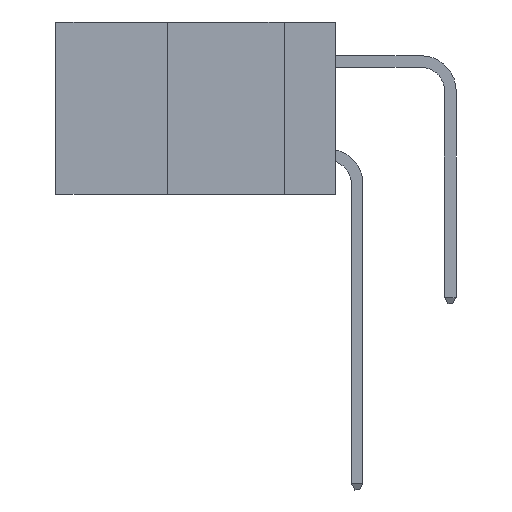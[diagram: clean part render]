
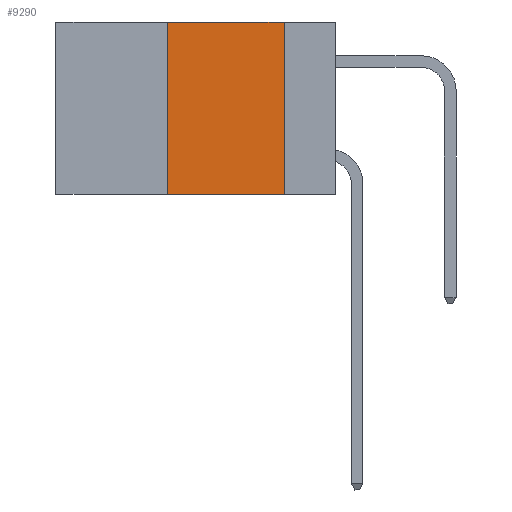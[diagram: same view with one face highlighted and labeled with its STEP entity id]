
A CAD part, left-side view. The second image highlights one B-rep face of the part: STEP entity #9290.
In plain terms, the highlighted planar face has unit normal (-1, 0, 0).
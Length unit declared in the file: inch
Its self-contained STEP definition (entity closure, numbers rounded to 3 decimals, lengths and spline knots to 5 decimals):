
#184 = ORIENTED_EDGE ( 'NONE', *, *, #9923, .F. ) ;
#198 = ORIENTED_EDGE ( 'NONE', *, *, #2164, .T. ) ;
#483 = CARTESIAN_POINT ( 'NONE',  ( 0., 0.36, -0.37 ) ) ;
#531 = LINE ( 'NONE', #1199, #10162 ) ;
#1199 = CARTESIAN_POINT ( 'NONE',  ( 0., 0.11, 0. ) ) ;
#1274 = DIRECTION ( 'NONE',  ( 0., 0., -1. ) ) ;
#1278 = VERTEX_POINT ( 'NONE', #7535 ) ;
#1319 = LINE ( 'NONE', #3607, #6776 ) ;
#1543 = DIRECTION ( 'NONE',  ( 1., 0., 0. ) ) ;
#1597 = EDGE_CURVE ( 'NONE', #6915, #7989, #531, .T. ) ;
#1694 = CARTESIAN_POINT ( 'NONE',  ( 0., 0.11, -0.37 ) ) ;
#2164 = EDGE_CURVE ( 'NONE', #4565, #7989, #7359, .T. ) ;
#2437 = VECTOR ( 'NONE', #5425, 39.37008 ) ;
#2674 = ORIENTED_EDGE ( 'NONE', *, *, #4798, .F. ) ;
#2956 = VECTOR ( 'NONE', #10733, 39.37008 ) ;
#3059 = CARTESIAN_POINT ( 'NONE',  ( 0., 0.6, 0. ) ) ;
#3607 = CARTESIAN_POINT ( 'NONE',  ( 0., 0.36, 0. ) ) ;
#4565 = VERTEX_POINT ( 'NONE', #483 ) ;
#4798 = EDGE_CURVE ( 'NONE', #1278, #6915, #9361, .T. ) ;
#5425 = DIRECTION ( 'NONE',  ( 0., -1., 0. ) ) ;
#6776 = VECTOR ( 'NONE', #7130, 39.37008 ) ;
#6915 = VERTEX_POINT ( 'NONE', #11232 ) ;
#7004 = CARTESIAN_POINT ( 'NONE',  ( 0., 0.6, 0. ) ) ;
#7130 = DIRECTION ( 'NONE',  ( 0., 0., 1. ) ) ;
#7359 = LINE ( 'NONE', #10716, #2956 ) ;
#7491 = EDGE_LOOP ( 'NONE', ( #9101, #2674, #184, #198 ) ) ;
#7535 = CARTESIAN_POINT ( 'NONE',  ( 0., 0.36, 0. ) ) ;
#7850 = DIRECTION ( 'NONE',  ( 0., 0., -1. ) ) ;
#7989 = VERTEX_POINT ( 'NONE', #1694 ) ;
#8117 = FACE_OUTER_BOUND ( 'NONE', #7491, .T. ) ;
#9101 = ORIENTED_EDGE ( 'NONE', *, *, #1597, .F. ) ;
#9290 = ADVANCED_FACE ( 'NONE', ( #8117 ), #11034, .F. ) ;
#9361 = LINE ( 'NONE', #3059, #2437 ) ;
#9923 = EDGE_CURVE ( 'NONE', #4565, #1278, #1319, .T. ) ;
#9988 = AXIS2_PLACEMENT_3D ( 'NONE', #7004, #1543, #7850 ) ;
#10162 = VECTOR ( 'NONE', #1274, 39.37008 ) ;
#10716 = CARTESIAN_POINT ( 'NONE',  ( 0., 0.6, -0.37 ) ) ;
#10733 = DIRECTION ( 'NONE',  ( 0., -1., 0. ) ) ;
#11034 = PLANE ( 'NONE',  #9988 ) ;
#11232 = CARTESIAN_POINT ( 'NONE',  ( 0., 0.11, 0. ) ) ;
